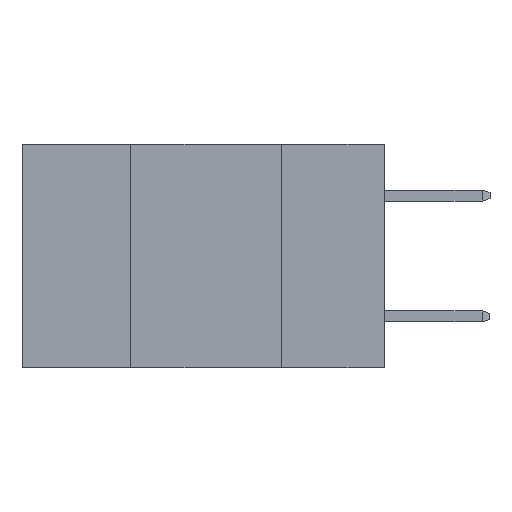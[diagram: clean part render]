
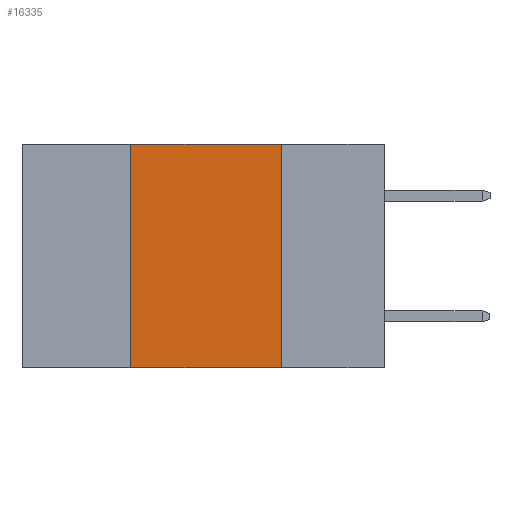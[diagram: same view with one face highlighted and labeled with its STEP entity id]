
A CAD part, left-side view. The second image highlights one B-rep face of the part: STEP entity #16335.
In plain terms, the highlighted planar face has unit normal (-1, 0, 0).
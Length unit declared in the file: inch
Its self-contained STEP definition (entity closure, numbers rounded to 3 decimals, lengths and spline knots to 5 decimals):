
#80 = EDGE_CURVE ( 'NONE', #4705, #15121, #15484, .T. ) ;
#1639 = CARTESIAN_POINT ( 'NONE',  ( 0., 0.42, 0. ) ) ;
#2405 = CARTESIAN_POINT ( 'NONE',  ( 0., 0.6, 0. ) ) ;
#3498 = VECTOR ( 'NONE', #12529, 39.37008 ) ;
#3672 = VECTOR ( 'NONE', #18680, 39.37008 ) ;
#3738 = VECTOR ( 'NONE', #26994, 39.37008 ) ;
#3957 = EDGE_CURVE ( 'NONE', #7614, #15121, #28820, .T. ) ;
#4705 = VERTEX_POINT ( 'NONE', #26265 ) ;
#5238 = CARTESIAN_POINT ( 'NONE',  ( 0., 0.17, -0.37 ) ) ;
#5417 = DIRECTION ( 'NONE',  ( 0., -1., 0. ) ) ;
#7454 = FACE_OUTER_BOUND ( 'NONE', #24953, .T. ) ;
#7575 = CARTESIAN_POINT ( 'NONE',  ( 0., 0.6, 0. ) ) ;
#7614 = VERTEX_POINT ( 'NONE', #20004 ) ;
#9467 = EDGE_CURVE ( 'NONE', #4705, #14830, #9969, .T. ) ;
#9756 = DIRECTION ( 'NONE',  ( 1., 0., 0. ) ) ;
#9969 = LINE ( 'NONE', #24745, #3498 ) ;
#12056 = EDGE_CURVE ( 'NONE', #14830, #7614, #30372, .T. ) ;
#12529 = DIRECTION ( 'NONE',  ( 0., 0., 1. ) ) ;
#14830 = VERTEX_POINT ( 'NONE', #1639 ) ;
#15121 = VERTEX_POINT ( 'NONE', #5238 ) ;
#15484 = LINE ( 'NONE', #17655, #17028 ) ;
#16335 = ADVANCED_FACE ( 'NONE', ( #7454 ), #24388, .F. ) ;
#16364 = ORIENTED_EDGE ( 'NONE', *, *, #9467, .F. ) ;
#17028 = VECTOR ( 'NONE', #5417, 39.37008 ) ;
#17655 = CARTESIAN_POINT ( 'NONE',  ( 0., 0.6, -0.37 ) ) ;
#17769 = ORIENTED_EDGE ( 'NONE', *, *, #3957, .F. ) ;
#18285 = ORIENTED_EDGE ( 'NONE', *, *, #80, .T. ) ;
#18680 = DIRECTION ( 'NONE',  ( 0., 0., -1. ) ) ;
#19822 = AXIS2_PLACEMENT_3D ( 'NONE', #2405, #9756, #26847 ) ;
#20004 = CARTESIAN_POINT ( 'NONE',  ( 0., 0.17, 0. ) ) ;
#24388 = PLANE ( 'NONE',  #19822 ) ;
#24745 = CARTESIAN_POINT ( 'NONE',  ( 0., 0.42, 0. ) ) ;
#24953 = EDGE_LOOP ( 'NONE', ( #17769, #29140, #16364, #18285 ) ) ;
#26265 = CARTESIAN_POINT ( 'NONE',  ( 0., 0.42, -0.37 ) ) ;
#26847 = DIRECTION ( 'NONE',  ( 0., 0., -1. ) ) ;
#26994 = DIRECTION ( 'NONE',  ( 0., -1., 0. ) ) ;
#28820 = LINE ( 'NONE', #29394, #3672 ) ;
#29140 = ORIENTED_EDGE ( 'NONE', *, *, #12056, .F. ) ;
#29394 = CARTESIAN_POINT ( 'NONE',  ( 0., 0.17, 0. ) ) ;
#30372 = LINE ( 'NONE', #7575, #3738 ) ;
